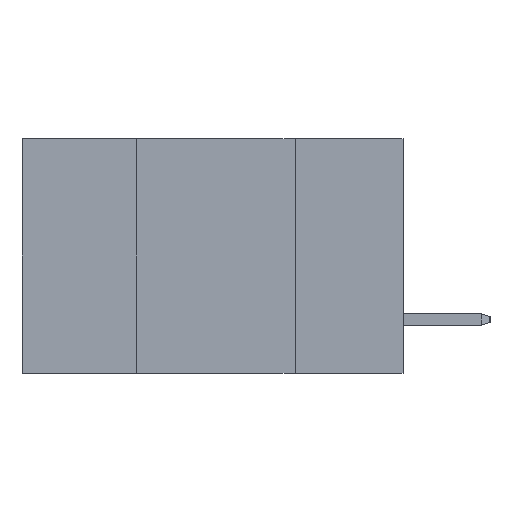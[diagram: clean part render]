
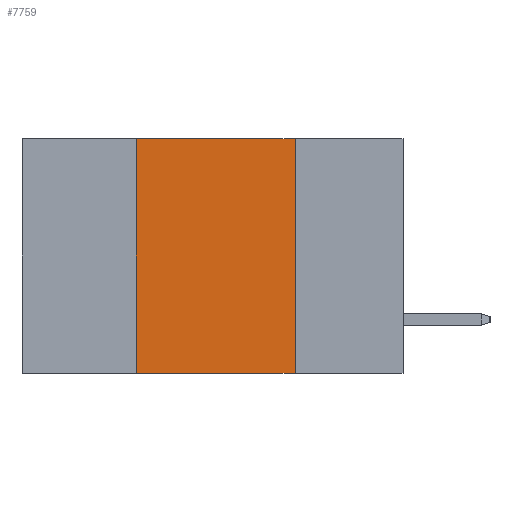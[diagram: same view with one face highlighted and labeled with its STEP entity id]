
A CAD part, left-side view. The second image highlights one B-rep face of the part: STEP entity #7759.
In plain terms, the highlighted planar face has unit normal (-1, 0, 0).
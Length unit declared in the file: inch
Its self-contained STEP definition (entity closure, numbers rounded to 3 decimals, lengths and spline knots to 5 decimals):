
#35 = VECTOR ( 'NONE', #9504, 39.37008 ) ;
#51 = VECTOR ( 'NONE', #7289, 39.37008 ) ;
#139 = CARTESIAN_POINT ( 'NONE',  ( 0., 0.6, 0. ) ) ;
#143 = ORIENTED_EDGE ( 'NONE', *, *, #3691, .T. ) ;
#333 = LINE ( 'NONE', #4011, #7775 ) ;
#840 = EDGE_CURVE ( 'NONE', #1411, #8384, #3456, .T. ) ;
#1411 = VERTEX_POINT ( 'NONE', #6664 ) ;
#1840 = DIRECTION ( 'NONE',  ( 0., 0., -1. ) ) ;
#2152 = EDGE_LOOP ( 'NONE', ( #8760, #5980, #2702, #143 ) ) ;
#2702 = ORIENTED_EDGE ( 'NONE', *, *, #4591, .F. ) ;
#3054 = PLANE ( 'NONE',  #4098 ) ;
#3446 = LINE ( 'NONE', #7263, #35 ) ;
#3456 = LINE ( 'NONE', #6411, #7419 ) ;
#3691 = EDGE_CURVE ( 'NONE', #4684, #8768, #3446, .T. ) ;
#4011 = CARTESIAN_POINT ( 'NONE',  ( 0., 0.17, 0. ) ) ;
#4098 = AXIS2_PLACEMENT_3D ( 'NONE', #139, #6048, #9011 ) ;
#4149 = LINE ( 'NONE', #8704, #51 ) ;
#4237 = DIRECTION ( 'NONE',  ( 0., -1., 0. ) ) ;
#4591 = EDGE_CURVE ( 'NONE', #4684, #1411, #4149, .T. ) ;
#4684 = VERTEX_POINT ( 'NONE', #8070 ) ;
#5273 = FACE_OUTER_BOUND ( 'NONE', #2152, .T. ) ;
#5660 = EDGE_CURVE ( 'NONE', #8384, #8768, #333, .T. ) ;
#5980 = ORIENTED_EDGE ( 'NONE', *, *, #840, .F. ) ;
#6048 = DIRECTION ( 'NONE',  ( 1., 0., 0. ) ) ;
#6316 = CARTESIAN_POINT ( 'NONE',  ( 0., 0.17, 0. ) ) ;
#6411 = CARTESIAN_POINT ( 'NONE',  ( 0., 0.6, 0. ) ) ;
#6664 = CARTESIAN_POINT ( 'NONE',  ( 0., 0.42, 0. ) ) ;
#7263 = CARTESIAN_POINT ( 'NONE',  ( 0., 0.6, -0.37 ) ) ;
#7289 = DIRECTION ( 'NONE',  ( 0., 0., 1. ) ) ;
#7419 = VECTOR ( 'NONE', #4237, 39.37008 ) ;
#7759 = ADVANCED_FACE ( 'NONE', ( #5273 ), #3054, .F. ) ;
#7775 = VECTOR ( 'NONE', #1840, 39.37008 ) ;
#8070 = CARTESIAN_POINT ( 'NONE',  ( 0., 0.42, -0.37 ) ) ;
#8302 = CARTESIAN_POINT ( 'NONE',  ( 0., 0.17, -0.37 ) ) ;
#8384 = VERTEX_POINT ( 'NONE', #6316 ) ;
#8704 = CARTESIAN_POINT ( 'NONE',  ( 0., 0.42, 0. ) ) ;
#8760 = ORIENTED_EDGE ( 'NONE', *, *, #5660, .F. ) ;
#8768 = VERTEX_POINT ( 'NONE', #8302 ) ;
#9011 = DIRECTION ( 'NONE',  ( 0., 0., -1. ) ) ;
#9504 = DIRECTION ( 'NONE',  ( 0., -1., 0. ) ) ;
